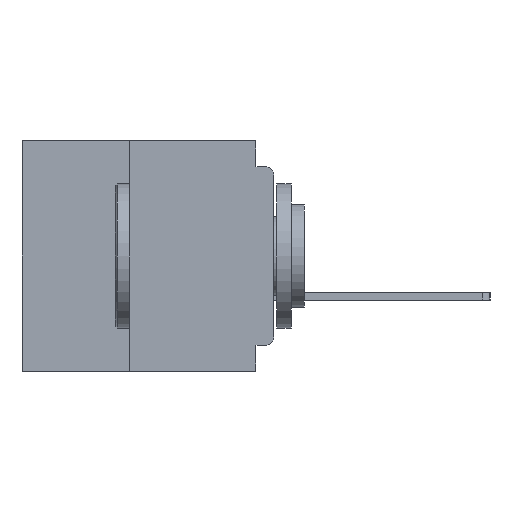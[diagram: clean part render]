
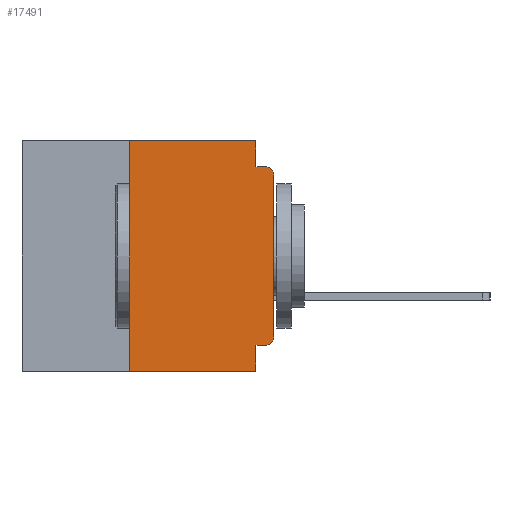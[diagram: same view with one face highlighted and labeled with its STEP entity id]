
A CAD part, left-side view. The second image highlights one B-rep face of the part: STEP entity #17491.
In plain terms, the highlighted planar face has unit normal (-1, 0, 0).
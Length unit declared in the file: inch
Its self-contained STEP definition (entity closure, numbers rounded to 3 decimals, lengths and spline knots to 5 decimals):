
#1624 = CARTESIAN_POINT ( 'NONE',  ( 0., 0., 0. ) ) ;
#2178 = DIRECTION ( 'NONE',  ( 0., -1., 0. ) ) ;
#2220 = VERTEX_POINT ( 'NONE', #57012 ) ;
#2732 = DIRECTION ( 'NONE',  ( 0., 0., -1. ) ) ;
#3150 = PLANE ( 'NONE',  #36441 ) ;
#4132 = DIRECTION ( 'NONE',  ( -1., 0., 0. ) ) ;
#4796 = VECTOR ( 'NONE', #21173, 39.37008 ) ;
#5585 = ORIENTED_EDGE ( 'NONE', *, *, #27955, .T. ) ;
#5824 = CARTESIAN_POINT ( 'NONE',  ( 0., 0.437, -0.4 ) ) ;
#6685 = VERTEX_POINT ( 'NONE', #28872 ) ;
#7954 = VERTEX_POINT ( 'NONE', #23749 ) ;
#8170 = DIRECTION ( 'NONE',  ( 1., 0., 0. ) ) ;
#9854 = VERTEX_POINT ( 'NONE', #47662 ) ;
#11311 = LINE ( 'NONE', #1624, #24583 ) ;
#11624 = LINE ( 'NONE', #61420, #62549 ) ;
#11933 = ORIENTED_EDGE ( 'NONE', *, *, #28826, .T. ) ;
#12206 = EDGE_CURVE ( 'NONE', #7954, #30520, #58518, .T. ) ;
#13299 = CARTESIAN_POINT ( 'NONE',  ( 0., 0.031, 0. ) ) ;
#13389 = ORIENTED_EDGE ( 'NONE', *, *, #21478, .T. ) ;
#17021 = CARTESIAN_POINT ( 'NONE',  ( 0., 0.031, -0.4 ) ) ;
#17491 = ADVANCED_FACE ( 'NONE', ( #61502 ), #3150, .F. ) ;
#18432 = CARTESIAN_POINT ( 'NONE',  ( 0., 0.031, -0.355 ) ) ;
#18738 = ORIENTED_EDGE ( 'NONE', *, *, #57665, .F. ) ;
#19211 = EDGE_CURVE ( 'NONE', #30520, #50959, #35201, .T. ) ;
#21173 = DIRECTION ( 'NONE',  ( 0., 0., 1. ) ) ;
#21478 = EDGE_CURVE ( 'NONE', #50157, #50959, #45828, .T. ) ;
#21725 = DIRECTION ( 'NONE',  ( 0., 1., 0. ) ) ;
#22652 = ORIENTED_EDGE ( 'NONE', *, *, #53676, .F. ) ;
#23749 = CARTESIAN_POINT ( 'NONE',  ( 0., 0.015, -0.355 ) ) ;
#24118 = VECTOR ( 'NONE', #47988, 39.37008 ) ;
#24510 = CARTESIAN_POINT ( 'NONE',  ( 0., 0.015, -0.06 ) ) ;
#24583 = VECTOR ( 'NONE', #41431, 39.37008 ) ;
#26078 = EDGE_CURVE ( 'NONE', #47219, #2220, #38829, .T. ) ;
#27955 = EDGE_CURVE ( 'NONE', #7954, #32823, #44000, .T. ) ;
#28826 = EDGE_CURVE ( 'NONE', #47113, #9854, #30737, .T. ) ;
#28872 = CARTESIAN_POINT ( 'NONE',  ( 0., 0.25, 0. ) ) ;
#29468 = DIRECTION ( 'NONE',  ( 0., 0., -1. ) ) ;
#30520 = VERTEX_POINT ( 'NONE', #18432 ) ;
#30737 = CIRCLE ( 'NONE', #52214, 0.015 ) ;
#30956 = CARTESIAN_POINT ( 'NONE',  ( 0., 0.25, -0.4 ) ) ;
#32823 = VERTEX_POINT ( 'NONE', #41372 ) ;
#33556 = CARTESIAN_POINT ( 'NONE',  ( 0., 0.031, 0. ) ) ;
#33977 = CARTESIAN_POINT ( 'NONE',  ( 0., 0.015, -0.34 ) ) ;
#34832 = EDGE_CURVE ( 'NONE', #32823, #47113, #11311, .T. ) ;
#35201 = LINE ( 'NONE', #61946, #59738 ) ;
#36156 = ORIENTED_EDGE ( 'NONE', *, *, #58500, .F. ) ;
#36441 = AXIS2_PLACEMENT_3D ( 'NONE', #57492, #8170, #42908 ) ;
#36464 = CARTESIAN_POINT ( 'NONE',  ( 0., 0., -0.355 ) ) ;
#37924 = LINE ( 'NONE', #53262, #62429 ) ;
#38829 = LINE ( 'NONE', #13299, #24118 ) ;
#38919 = DIRECTION ( 'NONE',  ( 0., 0., -1. ) ) ;
#41372 = CARTESIAN_POINT ( 'NONE',  ( 0., 0., -0.34 ) ) ;
#41431 = DIRECTION ( 'NONE',  ( 0., 0., 1. ) ) ;
#42451 = ORIENTED_EDGE ( 'NONE', *, *, #19211, .F. ) ;
#42908 = DIRECTION ( 'NONE',  ( 0., 0., -1. ) ) ;
#44000 = CIRCLE ( 'NONE', #46013, 0.015 ) ;
#44278 = VECTOR ( 'NONE', #50266, 39.37008 ) ;
#45828 = LINE ( 'NONE', #5824, #44278 ) ;
#46013 = AXIS2_PLACEMENT_3D ( 'NONE', #33977, #4132, #38919 ) ;
#47030 = ORIENTED_EDGE ( 'NONE', *, *, #26078, .F. ) ;
#47113 = VERTEX_POINT ( 'NONE', #52086 ) ;
#47219 = VERTEX_POINT ( 'NONE', #33556 ) ;
#47662 = CARTESIAN_POINT ( 'NONE',  ( 0., 0.015, -0.045 ) ) ;
#47988 = DIRECTION ( 'NONE',  ( 0., 0., -1. ) ) ;
#49470 = ORIENTED_EDGE ( 'NONE', *, *, #34832, .T. ) ;
#50157 = VERTEX_POINT ( 'NONE', #51131 ) ;
#50266 = DIRECTION ( 'NONE',  ( 0., -1., 0. ) ) ;
#50959 = VERTEX_POINT ( 'NONE', #17021 ) ;
#51131 = CARTESIAN_POINT ( 'NONE',  ( 0., 0.25, -0.4 ) ) ;
#51533 = ORIENTED_EDGE ( 'NONE', *, *, #12206, .F. ) ;
#52086 = CARTESIAN_POINT ( 'NONE',  ( 0., 0., -0.06 ) ) ;
#52214 = AXIS2_PLACEMENT_3D ( 'NONE', #24510, #58940, #29468 ) ;
#53262 = CARTESIAN_POINT ( 'NONE',  ( 0., 0.437, 0. ) ) ;
#53676 = EDGE_CURVE ( 'NONE', #50157, #6685, #57481, .T. ) ;
#56997 = VECTOR ( 'NONE', #21725, 39.37008 ) ;
#57012 = CARTESIAN_POINT ( 'NONE',  ( 0., 0.031, -0.045 ) ) ;
#57481 = LINE ( 'NONE', #30956, #4796 ) ;
#57492 = CARTESIAN_POINT ( 'NONE',  ( 0., 0.437, 0. ) ) ;
#57665 = EDGE_CURVE ( 'NONE', #2220, #9854, #11624, .T. ) ;
#58158 = DIRECTION ( 'NONE',  ( 0., -1., 0. ) ) ;
#58500 = EDGE_CURVE ( 'NONE', #6685, #47219, #37924, .T. ) ;
#58518 = LINE ( 'NONE', #36464, #56997 ) ;
#58940 = DIRECTION ( 'NONE',  ( -1., 0., 0. ) ) ;
#59738 = VECTOR ( 'NONE', #2732, 39.37008 ) ;
#60073 = EDGE_LOOP ( 'NONE', ( #49470, #11933, #18738, #47030, #36156, #22652, #13389, #42451, #51533, #5585 ) ) ;
#61420 = CARTESIAN_POINT ( 'NONE',  ( 0., 0., -0.045 ) ) ;
#61502 = FACE_OUTER_BOUND ( 'NONE', #60073, .T. ) ;
#61946 = CARTESIAN_POINT ( 'NONE',  ( 0., 0.031, -0.4 ) ) ;
#62429 = VECTOR ( 'NONE', #58158, 39.37008 ) ;
#62549 = VECTOR ( 'NONE', #2178, 39.37008 ) ;
